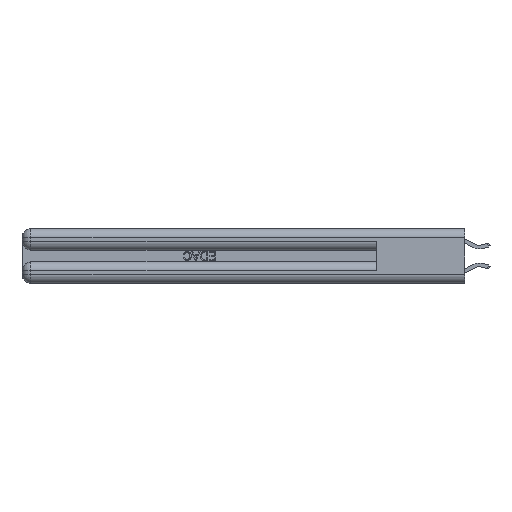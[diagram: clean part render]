
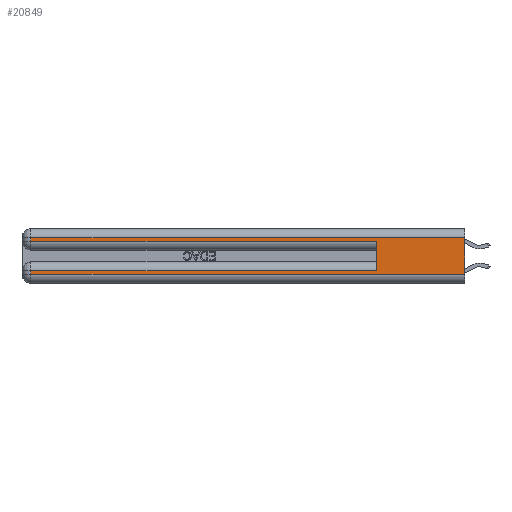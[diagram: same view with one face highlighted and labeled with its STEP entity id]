
A CAD part, left-side view. The second image highlights one B-rep face of the part: STEP entity #20849.
In plain terms, the highlighted planar face has unit normal (-1, 0, 0).
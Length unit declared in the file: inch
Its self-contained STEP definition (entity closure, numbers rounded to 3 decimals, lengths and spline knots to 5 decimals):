
#388 = CARTESIAN_POINT ( 'NONE',  ( 0., 0., 0.37 ) ) ;
#711 = EDGE_CURVE ( 'NONE', #24916, #19619, #11743, .T. ) ;
#851 = CARTESIAN_POINT ( 'NONE',  ( 0., 0., 0.37 ) ) ;
#1441 = CARTESIAN_POINT ( 'NONE',  ( 0., 2.94, 0.085 ) ) ;
#1596 = CARTESIAN_POINT ( 'NONE',  ( 0., 2.94, 0.06 ) ) ;
#2913 = VECTOR ( 'NONE', #31249, 39.37008 ) ;
#3015 = CARTESIAN_POINT ( 'NONE',  ( 0., 2.94, 0.285 ) ) ;
#3485 = DIRECTION ( 'NONE',  ( 0., 0., -1. ) ) ;
#4102 = VERTEX_POINT ( 'NONE', #24259 ) ;
#5111 = DIRECTION ( 'NONE',  ( 0., -1., 0. ) ) ;
#5568 = VECTOR ( 'NONE', #10688, 39.37008 ) ;
#6290 = VECTOR ( 'NONE', #6537, 39.37008 ) ;
#6537 = DIRECTION ( 'NONE',  ( 0., 1., 0. ) ) ;
#7250 = LINE ( 'NONE', #20873, #6290 ) ;
#7531 = VECTOR ( 'NONE', #5111, 39.37008 ) ;
#7801 = VERTEX_POINT ( 'NONE', #3015 ) ;
#8040 = EDGE_CURVE ( 'NONE', #32142, #15207, #21810, .T. ) ;
#8163 = ORIENTED_EDGE ( 'NONE', *, *, #711, .T. ) ;
#8399 = VERTEX_POINT ( 'NONE', #1441 ) ;
#8533 = EDGE_CURVE ( 'NONE', #4102, #33564, #27763, .T. ) ;
#9072 = LINE ( 'NONE', #29057, #2913 ) ;
#10688 = DIRECTION ( 'NONE',  ( 0., 0., 1. ) ) ;
#10947 = VECTOR ( 'NONE', #31007, 39.37008 ) ;
#11035 = CARTESIAN_POINT ( 'NONE',  ( 0., 0.6, 0.285 ) ) ;
#11177 = CARTESIAN_POINT ( 'NONE',  ( 0., 0., 0.285 ) ) ;
#11352 = LINE ( 'NONE', #11177, #22795 ) ;
#11573 = ORIENTED_EDGE ( 'NONE', *, *, #14679, .T. ) ;
#11743 = LINE ( 'NONE', #17380, #28956 ) ;
#12805 = LINE ( 'NONE', #23726, #23620 ) ;
#13542 = DIRECTION ( 'NONE',  ( 0., -1., 0. ) ) ;
#14679 = EDGE_CURVE ( 'NONE', #7801, #33564, #11352, .T. ) ;
#15002 = DIRECTION ( 'NONE',  ( 0., 0., -1. ) ) ;
#15207 = VERTEX_POINT ( 'NONE', #32776 ) ;
#15958 = EDGE_CURVE ( 'NONE', #4102, #8399, #7250, .T. ) ;
#17261 = FACE_OUTER_BOUND ( 'NONE', #35412, .T. ) ;
#17380 = CARTESIAN_POINT ( 'NONE',  ( 0., 0., 0.31 ) ) ;
#17720 = EDGE_CURVE ( 'NONE', #8399, #32142, #9072, .T. ) ;
#17731 = AXIS2_PLACEMENT_3D ( 'NONE', #388, #28359, #3485 ) ;
#17921 = ORIENTED_EDGE ( 'NONE', *, *, #32594, .T. ) ;
#19400 = LINE ( 'NONE', #851, #10947 ) ;
#19619 = VERTEX_POINT ( 'NONE', #23931 ) ;
#20545 = CARTESIAN_POINT ( 'NONE',  ( 0., 0., 0.31 ) ) ;
#20849 = ADVANCED_FACE ( 'NONE', ( #17261 ), #25292, .F. ) ;
#20873 = CARTESIAN_POINT ( 'NONE',  ( 0., 0., 0.085 ) ) ;
#21810 = LINE ( 'NONE', #29994, #7531 ) ;
#22326 = ORIENTED_EDGE ( 'NONE', *, *, #26426, .F. ) ;
#22795 = VECTOR ( 'NONE', #13542, 39.37008 ) ;
#23620 = VECTOR ( 'NONE', #15002, 39.37008 ) ;
#23726 = CARTESIAN_POINT ( 'NONE',  ( 0., 2.94, 0.37 ) ) ;
#23931 = CARTESIAN_POINT ( 'NONE',  ( 0., 2.94, 0.31 ) ) ;
#24259 = CARTESIAN_POINT ( 'NONE',  ( 0., 0.6, 0.085 ) ) ;
#24916 = VERTEX_POINT ( 'NONE', #20545 ) ;
#25229 = DIRECTION ( 'NONE',  ( 0., 1., 0. ) ) ;
#25292 = PLANE ( 'NONE',  #17731 ) ;
#26426 = EDGE_CURVE ( 'NONE', #24916, #15207, #19400, .T. ) ;
#27164 = ORIENTED_EDGE ( 'NONE', *, *, #17720, .T. ) ;
#27763 = LINE ( 'NONE', #33390, #5568 ) ;
#28359 = DIRECTION ( 'NONE',  ( 1., 0., 0. ) ) ;
#28956 = VECTOR ( 'NONE', #25229, 39.37008 ) ;
#29057 = CARTESIAN_POINT ( 'NONE',  ( 0., 2.94, 0.37 ) ) ;
#29994 = CARTESIAN_POINT ( 'NONE',  ( 0., 0., 0.06 ) ) ;
#31007 = DIRECTION ( 'NONE',  ( 0., 0., -1. ) ) ;
#31249 = DIRECTION ( 'NONE',  ( 0., 0., -1. ) ) ;
#32142 = VERTEX_POINT ( 'NONE', #1596 ) ;
#32407 = ORIENTED_EDGE ( 'NONE', *, *, #15958, .T. ) ;
#32594 = EDGE_CURVE ( 'NONE', #19619, #7801, #12805, .T. ) ;
#32776 = CARTESIAN_POINT ( 'NONE',  ( 0., 0., 0.06 ) ) ;
#33390 = CARTESIAN_POINT ( 'NONE',  ( 0., 0.6, 0.145 ) ) ;
#33564 = VERTEX_POINT ( 'NONE', #11035 ) ;
#34051 = ORIENTED_EDGE ( 'NONE', *, *, #8533, .F. ) ;
#35412 = EDGE_LOOP ( 'NONE', ( #22326, #8163, #17921, #11573, #34051, #32407, #27164, #35696 ) ) ;
#35696 = ORIENTED_EDGE ( 'NONE', *, *, #8040, .T. ) ;
